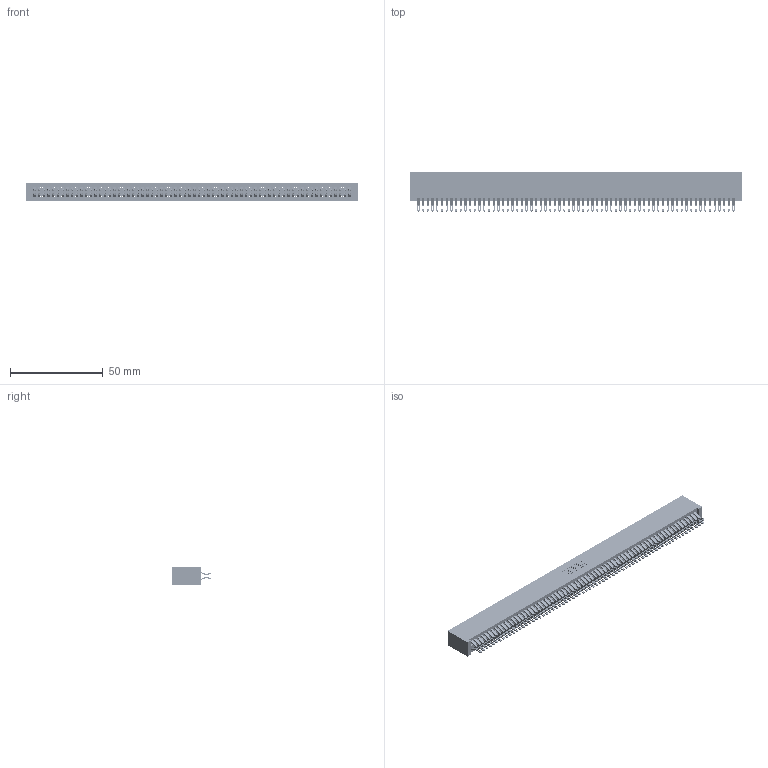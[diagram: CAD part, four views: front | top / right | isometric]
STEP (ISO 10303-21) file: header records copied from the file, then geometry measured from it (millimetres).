
FILE_DESCRIPTION (( 'STEP AP203' ), '1' );
FILE_NAME ('345-136-555-201.STEP', '2018-10-20T14:56:43', ( '' ), ( '' ), 'SwSTEP 2.0', 'SolidWorks 2016', '' );
FILE_SCHEMA (( 'CONFIG_CONTROL_DESIGN' ));
Length unit declared in the file: inch
Products named in the file (3): 345 Part_No Mounting Lugs; 345-292-001_555 Tail; 345-136-555-201
Assembly tree (137 placements, depth 2):
  345-136-555-201
    345 Part_No Mounting Lugs
    345-292-001_555 Tail  x136
Bounding box: 179.32 x 21.13 x 9.4 mm (x, y, z)
Volume: 18671.4 mm3; surface area: 29778.4 mm2
Topology: 137 solids, 137 shells, 7734 faces, 24389 edges, 16258 vertices
Faces by surface type: plane 4292, cylinder 3442
Entity records: 49903 total; most frequent: CARTESIAN_POINT 8374, ORIENTED_EDGE 8278, DIRECTION 7315, EDGE_CURVE 4139, VECTOR 3723, LINE 3723, VERTEX_POINT 2758, AXIS2_PLACEMENT_3D 1796
